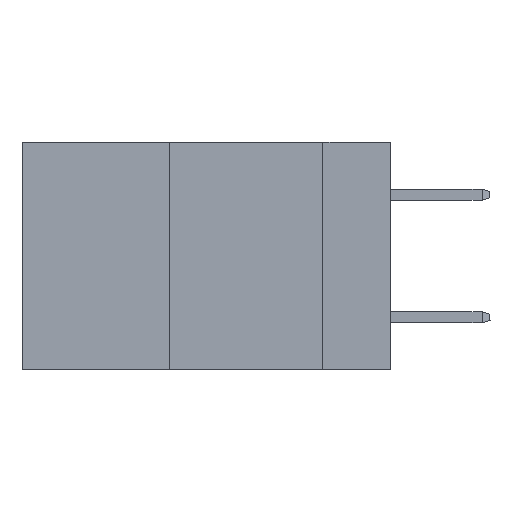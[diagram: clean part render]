
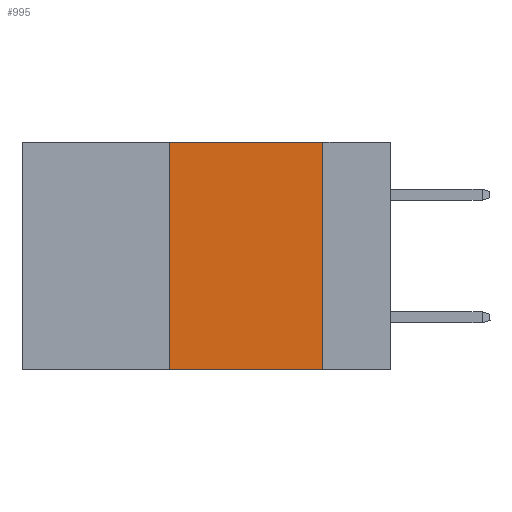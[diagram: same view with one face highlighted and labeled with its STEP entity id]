
A CAD part, left-side view. The second image highlights one B-rep face of the part: STEP entity #995.
In plain terms, the highlighted planar face has unit normal (-1, 0, 0).
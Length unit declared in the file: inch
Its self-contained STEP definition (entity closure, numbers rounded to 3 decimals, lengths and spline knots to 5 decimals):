
#202 = CARTESIAN_POINT ( 'NONE',  ( 0., 0.36, 0. ) ) ;
#973 = EDGE_CURVE ( 'NONE', #3423, #7230, #8504, .T. ) ;
#995 = ADVANCED_FACE ( 'NONE', ( #7654 ), #14415, .F. ) ;
#1504 = EDGE_LOOP ( 'NONE', ( #5871, #4386, #3265, #3471 ) ) ;
#1514 = VERTEX_POINT ( 'NONE', #3487 ) ;
#2905 = VECTOR ( 'NONE', #6706, 39.37008 ) ;
#3234 = VECTOR ( 'NONE', #5941, 39.37008 ) ;
#3265 = ORIENTED_EDGE ( 'NONE', *, *, #13046, .F. ) ;
#3423 = VERTEX_POINT ( 'NONE', #202 ) ;
#3471 = ORIENTED_EDGE ( 'NONE', *, *, #9500, .T. ) ;
#3487 = CARTESIAN_POINT ( 'NONE',  ( 0., 0.36, -0.37 ) ) ;
#3623 = VECTOR ( 'NONE', #16064, 39.37008 ) ;
#3915 = CARTESIAN_POINT ( 'NONE',  ( 0., 0.36, 0. ) ) ;
#4027 = AXIS2_PLACEMENT_3D ( 'NONE', #11762, #7798, #6440 ) ;
#4386 = ORIENTED_EDGE ( 'NONE', *, *, #973, .F. ) ;
#4557 = VERTEX_POINT ( 'NONE', #13599 ) ;
#4560 = CARTESIAN_POINT ( 'NONE',  ( 0., 0.11, 0. ) ) ;
#5871 = ORIENTED_EDGE ( 'NONE', *, *, #16215, .F. ) ;
#5941 = DIRECTION ( 'NONE',  ( 0., 0., -1. ) ) ;
#6440 = DIRECTION ( 'NONE',  ( 0., 0., -1. ) ) ;
#6629 = LINE ( 'NONE', #3915, #2905 ) ;
#6706 = DIRECTION ( 'NONE',  ( 0., 0., 1. ) ) ;
#6958 = LINE ( 'NONE', #4560, #3234 ) ;
#7230 = VERTEX_POINT ( 'NONE', #12617 ) ;
#7654 = FACE_OUTER_BOUND ( 'NONE', #1504, .T. ) ;
#7798 = DIRECTION ( 'NONE',  ( 1., 0., 0. ) ) ;
#8504 = LINE ( 'NONE', #12998, #14754 ) ;
#9500 = EDGE_CURVE ( 'NONE', #1514, #4557, #17479, .T. ) ;
#10445 = DIRECTION ( 'NONE',  ( 0., -1., 0. ) ) ;
#10777 = CARTESIAN_POINT ( 'NONE',  ( 0., 0.6, -0.37 ) ) ;
#11762 = CARTESIAN_POINT ( 'NONE',  ( 0., 0.6, 0. ) ) ;
#12617 = CARTESIAN_POINT ( 'NONE',  ( 0., 0.11, 0. ) ) ;
#12998 = CARTESIAN_POINT ( 'NONE',  ( 0., 0.6, 0. ) ) ;
#13046 = EDGE_CURVE ( 'NONE', #1514, #3423, #6629, .T. ) ;
#13599 = CARTESIAN_POINT ( 'NONE',  ( 0., 0.11, -0.37 ) ) ;
#14415 = PLANE ( 'NONE',  #4027 ) ;
#14754 = VECTOR ( 'NONE', #10445, 39.37008 ) ;
#16064 = DIRECTION ( 'NONE',  ( 0., -1., 0. ) ) ;
#16215 = EDGE_CURVE ( 'NONE', #7230, #4557, #6958, .T. ) ;
#17479 = LINE ( 'NONE', #10777, #3623 ) ;
